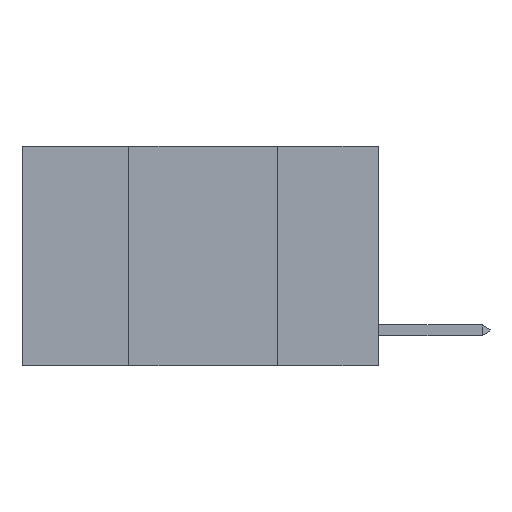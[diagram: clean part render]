
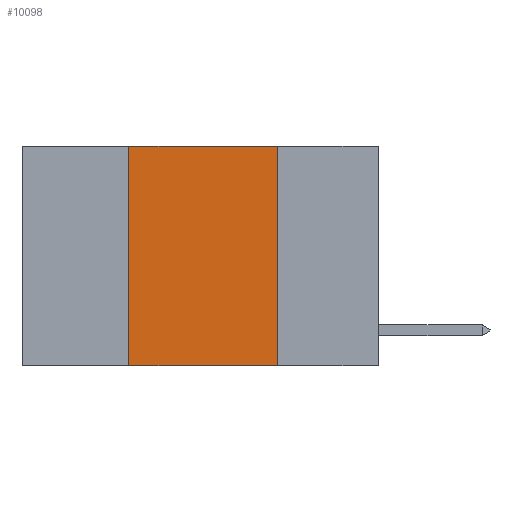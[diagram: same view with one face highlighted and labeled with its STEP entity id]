
A CAD part, left-side view. The second image highlights one B-rep face of the part: STEP entity #10098.
In plain terms, the highlighted planar face has unit normal (-1, 0, 0).
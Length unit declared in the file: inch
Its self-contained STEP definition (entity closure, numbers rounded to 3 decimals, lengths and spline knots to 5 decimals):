
#448 = VERTEX_POINT ( 'NONE', #1211 ) ;
#668 = LINE ( 'NONE', #5429, #8858 ) ;
#1211 = CARTESIAN_POINT ( 'NONE',  ( 0., 0.42, -0.37 ) ) ;
#1463 = CARTESIAN_POINT ( 'NONE',  ( 0., 0.6, -0.37 ) ) ;
#1518 = CARTESIAN_POINT ( 'NONE',  ( 0., 0.17, 0. ) ) ;
#1884 = ORIENTED_EDGE ( 'NONE', *, *, #6192, .F. ) ;
#2010 = CARTESIAN_POINT ( 'NONE',  ( 0., 0.6, 0. ) ) ;
#2555 = ORIENTED_EDGE ( 'NONE', *, *, #4564, .F. ) ;
#2881 = EDGE_CURVE ( 'NONE', #9751, #4497, #6102, .T. ) ;
#3263 = ORIENTED_EDGE ( 'NONE', *, *, #5291, .T. ) ;
#3775 = DIRECTION ( 'NONE',  ( 0., -1., 0. ) ) ;
#4069 = VECTOR ( 'NONE', #6520, 39.37008 ) ;
#4367 = VECTOR ( 'NONE', #4735, 39.37008 ) ;
#4497 = VERTEX_POINT ( 'NONE', #7633 ) ;
#4530 = CARTESIAN_POINT ( 'NONE',  ( 0., 0.17, 0. ) ) ;
#4564 = EDGE_CURVE ( 'NONE', #10055, #9751, #668, .T. ) ;
#4735 = DIRECTION ( 'NONE',  ( 0., 0., -1. ) ) ;
#5291 = EDGE_CURVE ( 'NONE', #448, #4497, #10361, .T. ) ;
#5429 = CARTESIAN_POINT ( 'NONE',  ( 0., 0.6, 0. ) ) ;
#6026 = AXIS2_PLACEMENT_3D ( 'NONE', #2010, #12195, #8219 ) ;
#6102 = LINE ( 'NONE', #4530, #4367 ) ;
#6192 = EDGE_CURVE ( 'NONE', #448, #10055, #9838, .T. ) ;
#6520 = DIRECTION ( 'NONE',  ( 0., 0., 1. ) ) ;
#7548 = DIRECTION ( 'NONE',  ( 0., -1., 0. ) ) ;
#7633 = CARTESIAN_POINT ( 'NONE',  ( 0., 0.17, -0.37 ) ) ;
#8022 = PLANE ( 'NONE',  #6026 ) ;
#8219 = DIRECTION ( 'NONE',  ( 0., 0., -1. ) ) ;
#8858 = VECTOR ( 'NONE', #3775, 39.37008 ) ;
#9446 = CARTESIAN_POINT ( 'NONE',  ( 0., 0.42, 0. ) ) ;
#9751 = VERTEX_POINT ( 'NONE', #1518 ) ;
#9807 = EDGE_LOOP ( 'NONE', ( #11908, #2555, #1884, #3263 ) ) ;
#9838 = LINE ( 'NONE', #9446, #4069 ) ;
#10055 = VERTEX_POINT ( 'NONE', #12009 ) ;
#10098 = ADVANCED_FACE ( 'NONE', ( #12794 ), #8022, .F. ) ;
#10361 = LINE ( 'NONE', #1463, #12368 ) ;
#11908 = ORIENTED_EDGE ( 'NONE', *, *, #2881, .F. ) ;
#12009 = CARTESIAN_POINT ( 'NONE',  ( 0., 0.42, 0. ) ) ;
#12195 = DIRECTION ( 'NONE',  ( 1., 0., 0. ) ) ;
#12368 = VECTOR ( 'NONE', #7548, 39.37008 ) ;
#12794 = FACE_OUTER_BOUND ( 'NONE', #9807, .T. ) ;
